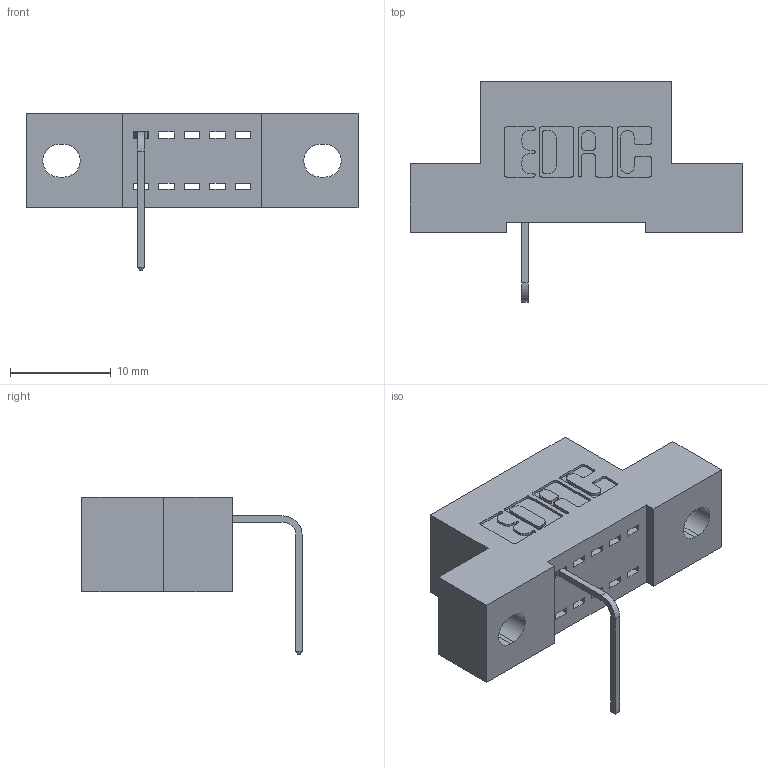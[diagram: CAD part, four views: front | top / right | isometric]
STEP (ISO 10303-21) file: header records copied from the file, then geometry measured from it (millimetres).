
FILE_DESCRIPTION (( 'STEP AP203' ), '1' );
FILE_NAME ('342-005-558-102.STEP', '2018-08-10T11:12:05', ( '' ), ( '' ), 'SwSTEP 2.0', 'SolidWorks 2016', '' );
FILE_SCHEMA (( 'CONFIG_CONTROL_DESIGN' ));
Length unit declared in the file: inch
Products named in the file (3): 342-005-558-102; 342 Part_.128 Slot; 345-292-001_558 Tail - 2
Assembly tree (2 placements, depth 2):
  342-005-558-102
    342 Part_.128 Slot
    345-292-001_558 Tail - 2
Bounding box: 33.02 x 21.91 x 15.62 mm (x, y, z)
Volume: 2664.4 mm3; surface area: 2763.1 mm2
Topology: 2 solids, 2 shells, 222 faces, 661 edges, 438 vertices
Faces by surface type: plane 162, cylinder 60
Entity records: 7801 total; most frequent: CARTESIAN_POINT 1377, ORIENTED_EDGE 1322, DIRECTION 1231, EDGE_CURVE 661, VECTOR 533, LINE 533, VERTEX_POINT 438, AXIS2_PLACEMENT_3D 349
